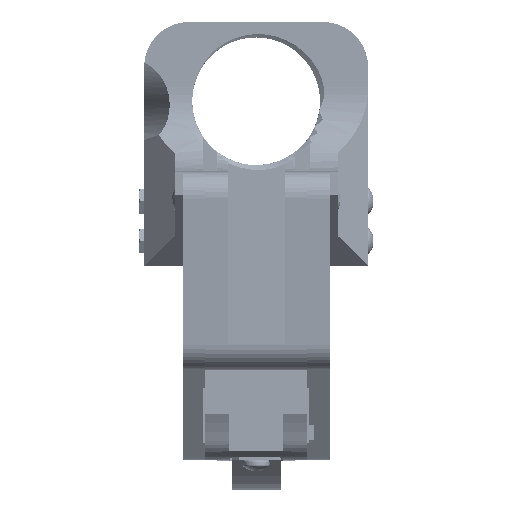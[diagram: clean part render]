
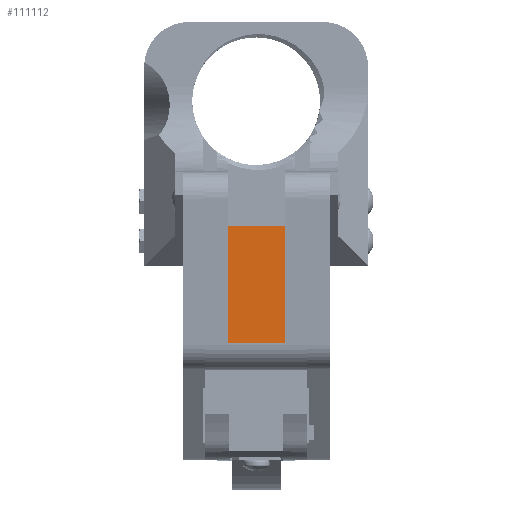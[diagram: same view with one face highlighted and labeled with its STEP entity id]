
A CAD part, top view. The second image highlights one B-rep face of the part: STEP entity #111112.
In plain terms, the highlighted face is planar.
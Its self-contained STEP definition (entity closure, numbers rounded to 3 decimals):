
#1070 = CARTESIAN_POINT ( 'NONE',  ( -33.027, -38.329, 2.5 ) ) ;
#2830 = CARTESIAN_POINT ( 'NONE',  ( -33.027, -38.329, 2.5 ) ) ;
#5042 = VERTEX_POINT ( 'NONE', #84464 ) ;
#6263 = LINE ( 'NONE', #2830, #81297 ) ;
#10343 = AXIS2_PLACEMENT_3D ( 'NONE', #1070, #89231, #30528 ) ;
#21818 = LINE ( 'NONE', #113600, #125901 ) ;
#26628 = ORIENTED_EDGE ( 'NONE', *, *, #48231, .F. ) ;
#28268 = LINE ( 'NONE', #45576, #103293 ) ;
#28364 = ORIENTED_EDGE ( 'NONE', *, *, #84492, .T. ) ;
#29024 = EDGE_CURVE ( 'NONE', #117198, #121400, #6263, .T. ) ;
#30528 = DIRECTION ( 'NONE',  ( 1., 0., 0. ) ) ;
#35714 = DIRECTION ( 'NONE',  ( 0., -1., 0. ) ) ;
#45576 = CARTESIAN_POINT ( 'NONE',  ( -6.35, -38.329, 2.5 ) ) ;
#45731 = LINE ( 'NONE', #88033, #48808 ) ;
#48231 = EDGE_CURVE ( 'NONE', #121400, #72021, #45731, .T. ) ;
#48808 = VECTOR ( 'NONE', #68393, 1000. ) ;
#52618 = EDGE_CURVE ( 'NONE', #5042, #117198, #28268, .T. ) ;
#53970 = CARTESIAN_POINT ( 'NONE',  ( -6.35, -38.329, 2.5 ) ) ;
#55041 = FACE_OUTER_BOUND ( 'NONE', #80942, .T. ) ;
#60377 = ORIENTED_EDGE ( 'NONE', *, *, #29024, .F. ) ;
#68393 = DIRECTION ( 'NONE',  ( 0., 1., 0. ) ) ;
#70583 = CARTESIAN_POINT ( 'NONE',  ( 6.35, -38.329, 2.5 ) ) ;
#71365 = DIRECTION ( 'NONE',  ( 1., 0., 0. ) ) ;
#72021 = VERTEX_POINT ( 'NONE', #120677 ) ;
#79409 = PLANE ( 'NONE',  #10343 ) ;
#80942 = EDGE_LOOP ( 'NONE', ( #28364, #26628, #60377, #114629 ) ) ;
#81297 = VECTOR ( 'NONE', #71365, 1000. ) ;
#84464 = CARTESIAN_POINT ( 'NONE',  ( -6.35, -12.192, 2.5 ) ) ;
#84492 = EDGE_CURVE ( 'NONE', #5042, #72021, #21818, .T. ) ;
#88033 = CARTESIAN_POINT ( 'NONE',  ( 6.35, -38.329, 2.5 ) ) ;
#89231 = DIRECTION ( 'NONE',  ( 0., 0., 1. ) ) ;
#93554 = DIRECTION ( 'NONE',  ( 1., 0., 0. ) ) ;
#103293 = VECTOR ( 'NONE', #35714, 1000. ) ;
#111112 = ADVANCED_FACE ( 'NONE', ( #55041 ), #79409, .F. ) ;
#113600 = CARTESIAN_POINT ( 'NONE',  ( -33.027, -12.192, 2.5 ) ) ;
#114629 = ORIENTED_EDGE ( 'NONE', *, *, #52618, .F. ) ;
#117198 = VERTEX_POINT ( 'NONE', #53970 ) ;
#120677 = CARTESIAN_POINT ( 'NONE',  ( 6.35, -12.192, 2.5 ) ) ;
#121400 = VERTEX_POINT ( 'NONE', #70583 ) ;
#125901 = VECTOR ( 'NONE', #93554, 1000. ) ;
